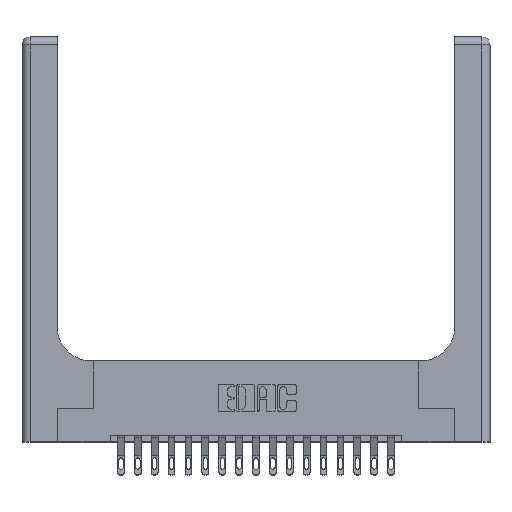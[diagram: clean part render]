
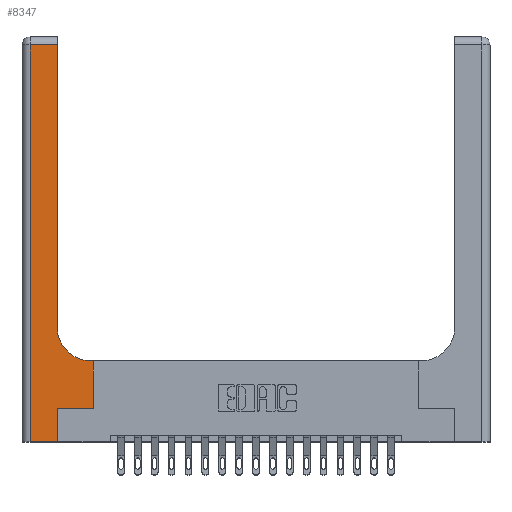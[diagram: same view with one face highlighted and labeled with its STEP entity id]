
A CAD part, top view. The second image highlights one B-rep face of the part: STEP entity #8347.
In plain terms, the highlighted planar face has unit normal (0, 0, 1).
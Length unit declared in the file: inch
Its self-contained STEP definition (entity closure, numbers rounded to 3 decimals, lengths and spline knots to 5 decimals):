
#563 = VECTOR ( 'NONE', #9222, 39.37008 ) ;
#710 = EDGE_CURVE ( 'NONE', #18824, #17992, #16316, .T. ) ;
#854 = CIRCLE ( 'NONE', #19925, 0.25 ) ;
#1088 = DIRECTION ( 'NONE',  ( 0., 1., 0. ) ) ;
#1109 = ORIENTED_EDGE ( 'NONE', *, *, #2421, .T. ) ;
#1312 = VECTOR ( 'NONE', #15093, 39.37008 ) ;
#1334 = CARTESIAN_POINT ( 'NONE',  ( 0.06, 3., 0.37 ) ) ;
#1373 = DIRECTION ( 'NONE',  ( 0., 0., -1. ) ) ;
#1975 = VERTEX_POINT ( 'NONE', #6364 ) ;
#2004 = DIRECTION ( 'NONE',  ( -1., 0., 0. ) ) ;
#2332 = CARTESIAN_POINT ( 'NONE',  ( 0.06, 0., 0.37 ) ) ;
#2345 = LINE ( 'NONE', #11375, #10364 ) ;
#2421 = EDGE_CURVE ( 'NONE', #11086, #18594, #7347, .T. ) ;
#3633 = ORIENTED_EDGE ( 'NONE', *, *, #4428, .T. ) ;
#4428 = EDGE_CURVE ( 'NONE', #1975, #12995, #9549, .T. ) ;
#4963 = VECTOR ( 'NONE', #10149, 39.37008 ) ;
#5306 = ORIENTED_EDGE ( 'NONE', *, *, #11891, .T. ) ;
#5641 = EDGE_CURVE ( 'NONE', #9799, #17687, #18396, .T. ) ;
#5888 = VECTOR ( 'NONE', #12677, 39.37008 ) ;
#6233 = PLANE ( 'NONE',  #10039 ) ;
#6364 = CARTESIAN_POINT ( 'NONE',  ( 0.265, 0.25, 0.37 ) ) ;
#7347 = LINE ( 'NONE', #8866, #1312 ) ;
#7812 = CARTESIAN_POINT ( 'NONE',  ( 0.26, 0.85, 0.37 ) ) ;
#8291 = CARTESIAN_POINT ( 'NONE',  ( 0.26, 2.94, 0.37 ) ) ;
#8347 = ADVANCED_FACE ( 'NONE', ( #9128 ), #6233, .F. ) ;
#8866 = CARTESIAN_POINT ( 'NONE',  ( 0.26, 0.6, 0.37 ) ) ;
#9128 = FACE_OUTER_BOUND ( 'NONE', #9945, .T. ) ;
#9222 = DIRECTION ( 'NONE',  ( 0., -1., 0. ) ) ;
#9540 = ORIENTED_EDGE ( 'NONE', *, *, #13825, .T. ) ;
#9549 = LINE ( 'NONE', #9667, #5888 ) ;
#9667 = CARTESIAN_POINT ( 'NONE',  ( 0.265, 0.25, 0.37 ) ) ;
#9798 = EDGE_CURVE ( 'NONE', #17992, #1975, #2345, .T. ) ;
#9799 = VERTEX_POINT ( 'NONE', #8291 ) ;
#9810 = DIRECTION ( 'NONE',  ( 0., 1., 0. ) ) ;
#9894 = DIRECTION ( 'NONE',  ( 0., 1., 0. ) ) ;
#9945 = EDGE_LOOP ( 'NONE', ( #16101, #11913, #5306, #12791, #14004, #3633, #9540, #1109, #15880 ) ) ;
#10039 = AXIS2_PLACEMENT_3D ( 'NONE', #17177, #17300, #2004 ) ;
#10058 = EDGE_CURVE ( 'NONE', #17070, #9799, #18985, .T. ) ;
#10149 = DIRECTION ( 'NONE',  ( 1., 0., 0. ) ) ;
#10346 = CARTESIAN_POINT ( 'NONE',  ( 0.528, 0.6, 0.37 ) ) ;
#10351 = CARTESIAN_POINT ( 'NONE',  ( 0.26, 3., 0.37 ) ) ;
#10364 = VECTOR ( 'NONE', #9810, 39.37008 ) ;
#10555 = CARTESIAN_POINT ( 'NONE',  ( 0.265, 0., 0.37 ) ) ;
#10628 = CARTESIAN_POINT ( 'NONE',  ( 0.528, 0.25, 0.37 ) ) ;
#11086 = VERTEX_POINT ( 'NONE', #10346 ) ;
#11375 = CARTESIAN_POINT ( 'NONE',  ( 0.265, 0., 0.37 ) ) ;
#11572 = CARTESIAN_POINT ( 'NONE',  ( 0., 0., 0.37 ) ) ;
#11891 = EDGE_CURVE ( 'NONE', #17687, #18824, #18656, .T. ) ;
#11913 = ORIENTED_EDGE ( 'NONE', *, *, #5641, .T. ) ;
#12677 = DIRECTION ( 'NONE',  ( 1., 0., 0. ) ) ;
#12791 = ORIENTED_EDGE ( 'NONE', *, *, #710, .T. ) ;
#12995 = VERTEX_POINT ( 'NONE', #10628 ) ;
#13004 = CARTESIAN_POINT ( 'NONE',  ( 0.06, 2.94, 0.37 ) ) ;
#13330 = LINE ( 'NONE', #19098, #15947 ) ;
#13696 = CARTESIAN_POINT ( 'NONE',  ( 0.51, 0.6, 0.37 ) ) ;
#13825 = EDGE_CURVE ( 'NONE', #12995, #11086, #13330, .T. ) ;
#14004 = ORIENTED_EDGE ( 'NONE', *, *, #9798, .T. ) ;
#15093 = DIRECTION ( 'NONE',  ( -1., 0., 0. ) ) ;
#15284 = DIRECTION ( 'NONE',  ( 1., 0., 0. ) ) ;
#15793 = VECTOR ( 'NONE', #17972, 39.37008 ) ;
#15880 = ORIENTED_EDGE ( 'NONE', *, *, #17440, .T. ) ;
#15947 = VECTOR ( 'NONE', #9894, 39.37008 ) ;
#16101 = ORIENTED_EDGE ( 'NONE', *, *, #10058, .T. ) ;
#16316 = LINE ( 'NONE', #11572, #4963 ) ;
#16579 = VECTOR ( 'NONE', #1088, 39.37008 ) ;
#17070 = VERTEX_POINT ( 'NONE', #7812 ) ;
#17177 = CARTESIAN_POINT ( 'NONE',  ( 0., 3., 0.37 ) ) ;
#17300 = DIRECTION ( 'NONE',  ( 0., 0., -1. ) ) ;
#17440 = EDGE_CURVE ( 'NONE', #18594, #17070, #854, .T. ) ;
#17687 = VERTEX_POINT ( 'NONE', #13004 ) ;
#17972 = DIRECTION ( 'NONE',  ( -1., 0., 0. ) ) ;
#17992 = VERTEX_POINT ( 'NONE', #10555 ) ;
#18396 = LINE ( 'NONE', #19665, #15793 ) ;
#18594 = VERTEX_POINT ( 'NONE', #13696 ) ;
#18656 = LINE ( 'NONE', #1334, #563 ) ;
#18824 = VERTEX_POINT ( 'NONE', #2332 ) ;
#18985 = LINE ( 'NONE', #10351, #16579 ) ;
#19098 = CARTESIAN_POINT ( 'NONE',  ( 0.528, 0.25, 0.37 ) ) ;
#19665 = CARTESIAN_POINT ( 'NONE',  ( 0., 2.94, 0.37 ) ) ;
#19845 = CARTESIAN_POINT ( 'NONE',  ( 0.51, 0.85, 0.37 ) ) ;
#19925 = AXIS2_PLACEMENT_3D ( 'NONE', #19845, #1373, #15284 ) ;
